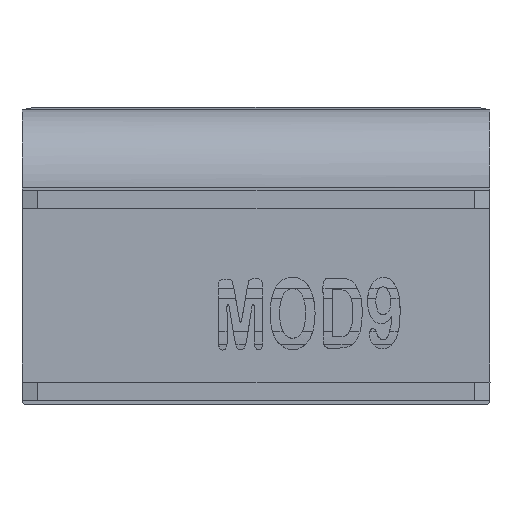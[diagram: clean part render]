
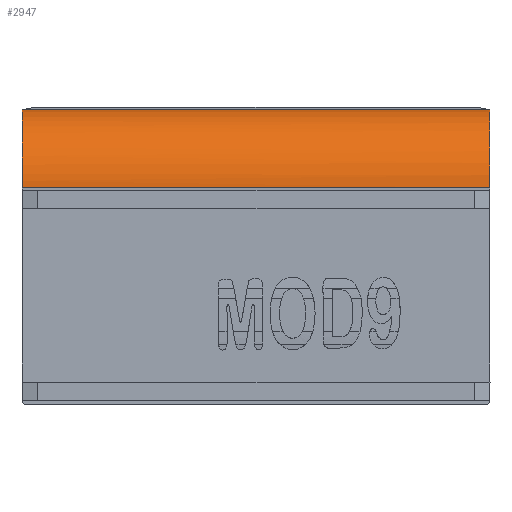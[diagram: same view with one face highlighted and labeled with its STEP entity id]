
A CAD part, top view. The second image highlights one B-rep face of the part: STEP entity #2947.
In plain terms, the highlighted cylindrical face has radius 13 mm (diameter 26 mm), a partial arc.
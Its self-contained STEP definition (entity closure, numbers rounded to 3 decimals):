
#284 = EDGE_CURVE ( 'NONE', #2779, #7553, #2871, .T. ) ;
#523 = CARTESIAN_POINT ( 'NONE',  ( -20.295, 60.808, 2.181 ) ) ;
#1068 = CARTESIAN_POINT ( 'NONE',  ( -46.024, 47.907, 13.681 ) ) ;
#1241 = ORIENTED_EDGE ( 'NONE', *, *, #284, .T. ) ;
#2543 = VECTOR ( 'NONE', #7879, 1000. ) ;
#2595 = EDGE_LOOP ( 'NONE', ( #9399, #9297, #5857, #1241 ) ) ;
#2779 = VERTEX_POINT ( 'NONE', #3361 ) ;
#2871 = B_SPLINE_CURVE_WITH_KNOTS ( 'NONE', 3,
 ( #8223, #9467, #11913, #8557, #3029, #10032, #6670, #4852, #11975, #3650 ),
 .UNSPECIFIED., .F., .F.,
 ( 4, 2, 2, 2, 4 ),
 ( 0., 0.25, 0.5, 0.75, 1. ),
 .UNSPECIFIED. ) ;
#2947 = ADVANCED_FACE ( 'NONE', ( #5838 ), #6741, .T. ) ;
#3029 = CARTESIAN_POINT ( 'NONE',  ( -97.484, 57.721, 9.337 ) ) ;
#3361 = CARTESIAN_POINT ( 'NONE',  ( -97.484, 60.808, 2.181 ) ) ;
#3614 = VERTEX_POINT ( 'NONE', #3808 ) ;
#3620 = CARTESIAN_POINT ( 'NONE',  ( -20.295, 47.907, 13.681 ) ) ;
#3650 = CARTESIAN_POINT ( 'NONE',  ( -97.484, 47.907, 13.681 ) ) ;
#3808 = CARTESIAN_POINT ( 'NONE',  ( -20.295, 60.808, 2.181 ) ) ;
#3911 = CARTESIAN_POINT ( 'NONE',  ( -20.295, 47.895, 0.681 ) ) ;
#4778 = CARTESIAN_POINT ( 'NONE',  ( -20.295, 47.907, 13.681 ) ) ;
#4852 = CARTESIAN_POINT ( 'NONE',  ( -97.484, 51.057, 13.389 ) ) ;
#5838 = FACE_OUTER_BOUND ( 'NONE', #2595, .T. ) ;
#5857 = ORIENTED_EDGE ( 'NONE', *, *, #9052, .T. ) ;
#6226 = LINE ( 'NONE', #523, #2543 ) ;
#6416 = CARTESIAN_POINT ( 'NONE',  ( -97.484, 47.907, 13.681 ) ) ;
#6670 = CARTESIAN_POINT ( 'NONE',  ( -97.484, 54.001, 12.265 ) ) ;
#6741 = CYLINDRICAL_SURFACE ( 'NONE', #8878, 13. ) ;
#6827 = VERTEX_POINT ( 'NONE', #4778 ) ;
#7120 = B_SPLINE_CURVE_WITH_KNOTS ( 'NONE', 3,
 ( #6416, #8253, #1068, #3620 ),
 .UNSPECIFIED., .F., .F.,
 ( 4, 4 ),
 ( 0., 1. ),
 .UNSPECIFIED. ) ;
#7319 = EDGE_CURVE ( 'NONE', #3614, #6827, #11843, .T. ) ;
#7553 = VERTEX_POINT ( 'NONE', #9124 ) ;
#7627 = DIRECTION ( 'NONE',  ( 0., 0., -1. ) ) ;
#7879 = DIRECTION ( 'NONE',  ( -1., 0., 0. ) ) ;
#8223 = CARTESIAN_POINT ( 'NONE',  ( -97.484, 60.808, 2.181 ) ) ;
#8253 = CARTESIAN_POINT ( 'NONE',  ( -71.754, 47.907, 13.681 ) ) ;
#8557 = CARTESIAN_POINT ( 'NONE',  ( -97.484, 58.704, 8.073 ) ) ;
#8574 = CARTESIAN_POINT ( 'NONE',  ( -20.295, 47.895, 0.681 ) ) ;
#8878 = AXIS2_PLACEMENT_3D ( 'NONE', #8574, #10636, #10517 ) ;
#9052 = EDGE_CURVE ( 'NONE', #3614, #2779, #6226, .T. ) ;
#9124 = CARTESIAN_POINT ( 'NONE',  ( -97.484, 47.907, 13.681 ) ) ;
#9297 = ORIENTED_EDGE ( 'NONE', *, *, #7319, .F. ) ;
#9315 = AXIS2_PLACEMENT_3D ( 'NONE', #3911, #10469, #7627 ) ;
#9399 = ORIENTED_EDGE ( 'NONE', *, *, #11348, .T. ) ;
#9467 = CARTESIAN_POINT ( 'NONE',  ( -97.484, 60.626, 3.746 ) ) ;
#10032 = CARTESIAN_POINT ( 'NONE',  ( -97.484, 55.369, 11.434 ) ) ;
#10469 = DIRECTION ( 'NONE',  ( 1., 0., 0. ) ) ;
#10517 = DIRECTION ( 'NONE',  ( 0., 0., -1. ) ) ;
#10636 = DIRECTION ( 'NONE',  ( 1., 0., 0. ) ) ;
#11348 = EDGE_CURVE ( 'NONE', #7553, #6827, #7120, .T. ) ;
#11843 = CIRCLE ( 'NONE', #9315, 13. ) ;
#11913 = CARTESIAN_POINT ( 'NONE',  ( -97.484, 60.157, 5.277 ) ) ;
#11975 = CARTESIAN_POINT ( 'NONE',  ( -97.484, 49.482, 13.68 ) ) ;
